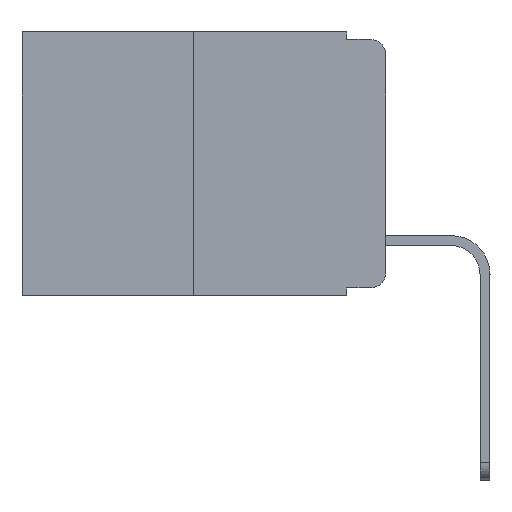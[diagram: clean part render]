
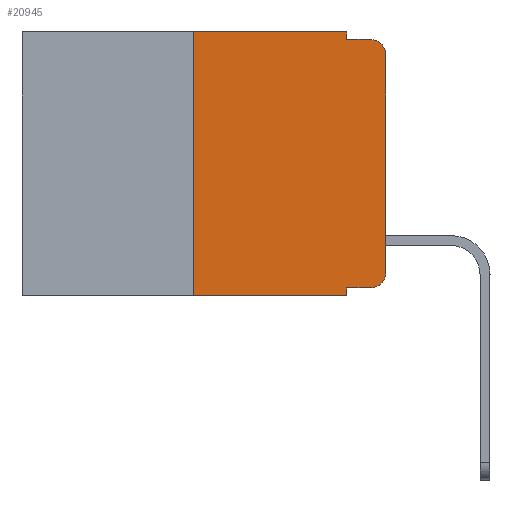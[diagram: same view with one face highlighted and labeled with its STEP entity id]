
A CAD part, left-side view. The second image highlights one B-rep face of the part: STEP entity #20945.
In plain terms, the highlighted planar face has unit normal (-1, 0, 0).
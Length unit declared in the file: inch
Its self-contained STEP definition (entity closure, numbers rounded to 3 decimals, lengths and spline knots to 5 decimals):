
#30 = DIRECTION ( 'NONE',  ( -1., 0., 0. ) ) ;
#31 = CARTESIAN_POINT ( 'NONE',  ( 0., 0.051, 0. ) ) ;
#45 = CARTESIAN_POINT ( 'NONE',  ( 0., 0.051, 0. ) ) ;
#786 = CARTESIAN_POINT ( 'NONE',  ( 0., 0.02, -0.313 ) ) ;
#1131 = DIRECTION ( 'NONE',  ( 0., 0., 1. ) ) ;
#1880 = EDGE_CURVE ( 'NONE', #6023, #14926, #4918, .T. ) ;
#1882 = ORIENTED_EDGE ( 'NONE', *, *, #8843, .F. ) ;
#2960 = EDGE_CURVE ( 'NONE', #11859, #18314, #15789, .T. ) ;
#2991 = AXIS2_PLACEMENT_3D ( 'NONE', #14795, #30, #22471 ) ;
#3404 = CARTESIAN_POINT ( 'NONE',  ( 0., 0.051, 0. ) ) ;
#4292 = DIRECTION ( 'NONE',  ( 0., -1., 0. ) ) ;
#4617 = VECTOR ( 'NONE', #1131, 39.37008 ) ;
#4918 = LINE ( 'NONE', #14033, #4617 ) ;
#4947 = ORIENTED_EDGE ( 'NONE', *, *, #8803, .F. ) ;
#5091 = EDGE_CURVE ( 'NONE', #8558, #15923, #17145, .T. ) ;
#5162 = LINE ( 'NONE', #22750, #7472 ) ;
#5453 = CARTESIAN_POINT ( 'NONE',  ( 0., 0.25, 0. ) ) ;
#5527 = VERTEX_POINT ( 'NONE', #11984 ) ;
#6023 = VERTEX_POINT ( 'NONE', #21165 ) ;
#6334 = LINE ( 'NONE', #3404, #17022 ) ;
#7147 = EDGE_CURVE ( 'NONE', #11859, #5527, #6334, .T. ) ;
#7196 = CIRCLE ( 'NONE', #2991, 0.02 ) ;
#7227 = DIRECTION ( 'NONE',  ( 0., 0., -1. ) ) ;
#7472 = VECTOR ( 'NONE', #15469, 39.37008 ) ;
#7946 = ORIENTED_EDGE ( 'NONE', *, *, #7147, .F. ) ;
#8215 = CARTESIAN_POINT ( 'NONE',  ( 0., 0.473, 0. ) ) ;
#8232 = DIRECTION ( 'NONE',  ( 0., -1., 0. ) ) ;
#8357 = DIRECTION ( 'NONE',  ( 0., 0., -1. ) ) ;
#8558 = VERTEX_POINT ( 'NONE', #16044 ) ;
#8697 = LINE ( 'NONE', #13167, #11238 ) ;
#8803 = EDGE_CURVE ( 'NONE', #17195, #22802, #18719, .T. ) ;
#8843 = EDGE_CURVE ( 'NONE', #21878, #8558, #14366, .T. ) ;
#9007 = DIRECTION ( 'NONE',  ( 0., 0., -1. ) ) ;
#9386 = ORIENTED_EDGE ( 'NONE', *, *, #1880, .T. ) ;
#11238 = VECTOR ( 'NONE', #4292, 39.37008 ) ;
#11623 = CIRCLE ( 'NONE', #12023, 0.02 ) ;
#11859 = VERTEX_POINT ( 'NONE', #22155 ) ;
#11951 = AXIS2_PLACEMENT_3D ( 'NONE', #8215, #23274, #8357 ) ;
#11984 = CARTESIAN_POINT ( 'NONE',  ( 0., 0.051, -0.343 ) ) ;
#12023 = AXIS2_PLACEMENT_3D ( 'NONE', #786, #19370, #13944 ) ;
#12097 = EDGE_LOOP ( 'NONE', ( #9386, #16039, #13404, #1882, #17425, #4947, #22413, #7946, #18104, #19870 ) ) ;
#12428 = CARTESIAN_POINT ( 'NONE',  ( 0., 0.25, -0.343 ) ) ;
#12502 = CARTESIAN_POINT ( 'NONE',  ( 0., 0.02, -0.333 ) ) ;
#12618 = VECTOR ( 'NONE', #9007, 39.37008 ) ;
#13167 = CARTESIAN_POINT ( 'NONE',  ( 0., 0.473, 0. ) ) ;
#13404 = ORIENTED_EDGE ( 'NONE', *, *, #5091, .F. ) ;
#13809 = EDGE_CURVE ( 'NONE', #14926, #15923, #7196, .T. ) ;
#13944 = DIRECTION ( 'NONE',  ( 0., 0., -1. ) ) ;
#14033 = CARTESIAN_POINT ( 'NONE',  ( 0., 0., 0. ) ) ;
#14366 = LINE ( 'NONE', #31, #12618 ) ;
#14475 = EDGE_CURVE ( 'NONE', #17195, #5527, #5162, .T. ) ;
#14639 = VECTOR ( 'NONE', #8232, 39.37008 ) ;
#14643 = CARTESIAN_POINT ( 'NONE',  ( 0., 0., -0.03 ) ) ;
#14795 = CARTESIAN_POINT ( 'NONE',  ( 0., 0.02, -0.03 ) ) ;
#14926 = VERTEX_POINT ( 'NONE', #14643 ) ;
#15469 = DIRECTION ( 'NONE',  ( 0., -1., 0. ) ) ;
#15716 = DIRECTION ( 'NONE',  ( 0., -1., 0. ) ) ;
#15789 = LINE ( 'NONE', #21504, #14639 ) ;
#15923 = VERTEX_POINT ( 'NONE', #18654 ) ;
#16039 = ORIENTED_EDGE ( 'NONE', *, *, #13809, .T. ) ;
#16044 = CARTESIAN_POINT ( 'NONE',  ( 0., 0.051, -0.01 ) ) ;
#16400 = EDGE_CURVE ( 'NONE', #18314, #6023, #11623, .T. ) ;
#17022 = VECTOR ( 'NONE', #7227, 39.37008 ) ;
#17145 = LINE ( 'NONE', #23384, #22703 ) ;
#17195 = VERTEX_POINT ( 'NONE', #12428 ) ;
#17425 = ORIENTED_EDGE ( 'NONE', *, *, #18053, .F. ) ;
#18053 = EDGE_CURVE ( 'NONE', #22802, #21878, #8697, .T. ) ;
#18104 = ORIENTED_EDGE ( 'NONE', *, *, #2960, .T. ) ;
#18314 = VERTEX_POINT ( 'NONE', #12502 ) ;
#18654 = CARTESIAN_POINT ( 'NONE',  ( 0., 0.02, -0.01 ) ) ;
#18719 = LINE ( 'NONE', #5453, #21352 ) ;
#19370 = DIRECTION ( 'NONE',  ( -1., 0., 0. ) ) ;
#19432 = PLANE ( 'NONE',  #11951 ) ;
#19870 = ORIENTED_EDGE ( 'NONE', *, *, #16400, .T. ) ;
#20481 = FACE_OUTER_BOUND ( 'NONE', #12097, .T. ) ;
#20945 = ADVANCED_FACE ( 'NONE', ( #20481 ), #19432, .F. ) ;
#21165 = CARTESIAN_POINT ( 'NONE',  ( 0., 0., -0.313 ) ) ;
#21352 = VECTOR ( 'NONE', #22069, 39.37008 ) ;
#21504 = CARTESIAN_POINT ( 'NONE',  ( 0., 0.051, -0.333 ) ) ;
#21732 = CARTESIAN_POINT ( 'NONE',  ( 0., 0.25, 0. ) ) ;
#21878 = VERTEX_POINT ( 'NONE', #45 ) ;
#22069 = DIRECTION ( 'NONE',  ( 0., 0., 1. ) ) ;
#22155 = CARTESIAN_POINT ( 'NONE',  ( 0., 0.051, -0.333 ) ) ;
#22413 = ORIENTED_EDGE ( 'NONE', *, *, #14475, .T. ) ;
#22471 = DIRECTION ( 'NONE',  ( 0., 0., -1. ) ) ;
#22703 = VECTOR ( 'NONE', #15716, 39.37008 ) ;
#22750 = CARTESIAN_POINT ( 'NONE',  ( 0., 0.473, -0.343 ) ) ;
#22802 = VERTEX_POINT ( 'NONE', #21732 ) ;
#23274 = DIRECTION ( 'NONE',  ( 1., 0., 0. ) ) ;
#23384 = CARTESIAN_POINT ( 'NONE',  ( 0., 0.051, -0.01 ) ) ;
